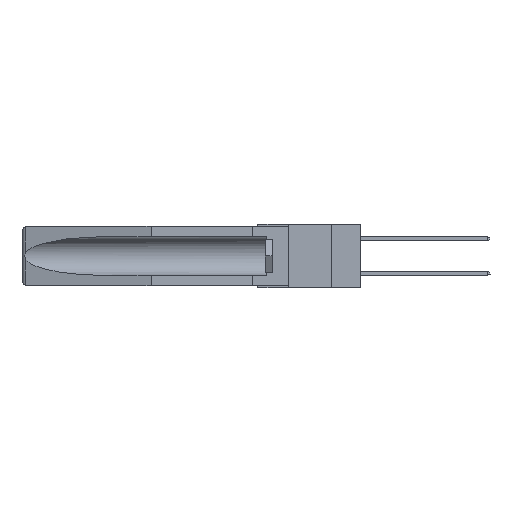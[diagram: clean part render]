
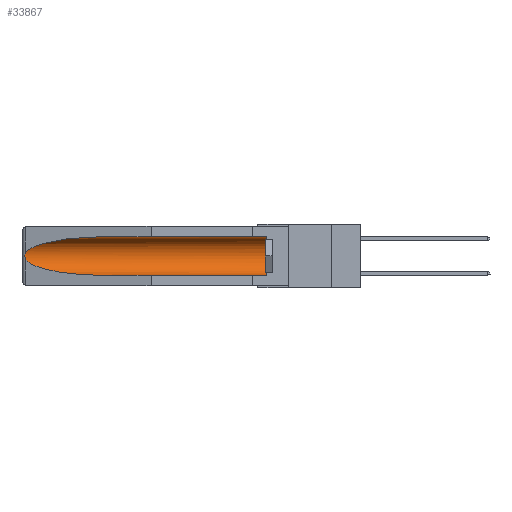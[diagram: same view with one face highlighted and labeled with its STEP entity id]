
A CAD part, left-side view. The second image highlights one B-rep face of the part: STEP entity #33867.
In plain terms, the highlighted cylindrical face has radius 2.857 mm (diameter 5.715 mm), a partial arc.
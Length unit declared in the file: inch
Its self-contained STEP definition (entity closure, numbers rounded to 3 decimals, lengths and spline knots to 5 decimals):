
#357 = ORIENTED_EDGE ( 'NONE', *, *, #7883, .T. ) ;
#951 = CARTESIAN_POINT ( 'NONE',  ( 0.26597, 1.5296, -0.19026 ) ) ;
#2775 = VERTEX_POINT ( 'NONE', #9192 ) ;
#3406 = EDGE_CURVE ( 'NONE', #28417, #9342, #11051, .T. ) ;
#3568 = CARTESIAN_POINT ( 'NONE',  ( 0.25451, 1.48313, -0.24835 ) ) ;
#3926 = DIRECTION ( 'NONE',  ( 0., 1., 0. ) ) ;
#4068 = ORIENTED_EDGE ( 'NONE', *, *, #5181, .T. ) ;
#4510 = AXIS2_PLACEMENT_3D ( 'NONE', #30480, #3926, #11827 ) ;
#4662 = CARTESIAN_POINT ( 'NONE',  ( 0.26537, 1.52718, -0.14972 ) ) ;
#5181 = EDGE_CURVE ( 'NONE', #28417, #31468, #23787, .T. ) ;
#6007 = DIRECTION ( 'NONE',  ( 0., 1., 0. ) ) ;
#6482 = CARTESIAN_POINT ( 'NONE',  ( 0.26537, 1.52718, -0.14972 ) ) ;
#6804 = CARTESIAN_POINT ( 'NONE',  ( 0.155, -0.30754, -0.284 ) ) ;
#7494 = FACE_OUTER_BOUND ( 'NONE', #24996, .T. ) ;
#7732 = ORIENTED_EDGE ( 'NONE', *, *, #31549, .T. ) ;
#7883 = EDGE_CURVE ( 'NONE', #24285, #2775, #11555, .T. ) ;
#8576 = CARTESIAN_POINT ( 'NONE',  ( 0.155, 0.126, -0.1715 ) ) ;
#9192 = CARTESIAN_POINT ( 'NONE',  ( 0.26537, 1.52718, -0.19328 ) ) ;
#9342 = VERTEX_POINT ( 'NONE', #11975 ) ;
#9935 = EDGE_CURVE ( 'NONE', #2775, #9342, #34099, .T. ) ;
#11051 = LINE ( 'NONE', #6804, #15234 ) ;
#11555 = B_SPLINE_CURVE_WITH_KNOTS ( 'NONE', 3,
 ( #6482, #22563, #30029, #14209, #14314, #32704, #19644, #16861, #951, #25066 ),
 .UNSPECIFIED., .F., .F.,
 ( 4, 2, 2, 2, 4 ),
 ( 0., 0.00029, 0.00058, 0.00087, 0.00117 ),
 .UNSPECIFIED. ) ;
#11804 = CARTESIAN_POINT ( 'NONE',  ( 0.26537, 1.52718, -0.19328 ) ) ;
#11827 = DIRECTION ( 'NONE',  ( 0., 0., 1. ) ) ;
#11975 = CARTESIAN_POINT ( 'NONE',  ( 0.155, 1.07973, -0.284 ) ) ;
#14209 = CARTESIAN_POINT ( 'NONE',  ( 0.2673, 1.5327, -0.16383 ) ) ;
#14314 = CARTESIAN_POINT ( 'NONE',  ( 0.2675, 1.53308, -0.16763 ) ) ;
#15201 =( BOUNDED_CURVE ( )  B_SPLINE_CURVE ( 3, ( #15371, #20609, #15599, #4662 ),
 .UNSPECIFIED., .F., .T. ) 
 B_SPLINE_CURVE_WITH_KNOTS ( ( 4, 4 ),
 ( 4.71239, 6.08839 ),
 .UNSPECIFIED. ) 
 CURVE ( )  GEOMETRIC_REPRESENTATION_ITEM ( )  RATIONAL_B_SPLINE_CURVE ( ( 1., 0.848, 0.848, 1. ) ) 
 REPRESENTATION_ITEM ( '' )  );
#15234 = VECTOR ( 'NONE', #19861, 39.37008 ) ;
#15371 = CARTESIAN_POINT ( 'NONE',  ( 0.155, 1.07973, -0.059 ) ) ;
#15599 = CARTESIAN_POINT ( 'NONE',  ( 0.25451, 1.48313, -0.09465 ) ) ;
#16861 = CARTESIAN_POINT ( 'NONE',  ( 0.26655, 1.53094, -0.18657 ) ) ;
#17263 = ORIENTED_EDGE ( 'NONE', *, *, #28318, .T. ) ;
#19644 = CARTESIAN_POINT ( 'NONE',  ( 0.2673, 1.53269, -0.17917 ) ) ;
#19861 = DIRECTION ( 'NONE',  ( 0., 1., 0. ) ) ;
#20609 = CARTESIAN_POINT ( 'NONE',  ( 0.21114, 1.30732, -0.059 ) ) ;
#20952 = LINE ( 'NONE', #27041, #21342 ) ;
#21342 = VECTOR ( 'NONE', #6007, 39.37008 ) ;
#21352 = ORIENTED_EDGE ( 'NONE', *, *, #9935, .T. ) ;
#22077 = DIRECTION ( 'NONE',  ( 0., 0., 1. ) ) ;
#22522 = CARTESIAN_POINT ( 'NONE',  ( 0.155, 1.07973, -0.284 ) ) ;
#22563 = CARTESIAN_POINT ( 'NONE',  ( 0.26597, 1.52961, -0.15275 ) ) ;
#23336 = AXIS2_PLACEMENT_3D ( 'NONE', #8576, #27131, #22077 ) ;
#23527 = CARTESIAN_POINT ( 'NONE',  ( 0.155, 1.07973, -0.059 ) ) ;
#23596 = CARTESIAN_POINT ( 'NONE',  ( 0.26537, 1.52718, -0.14972 ) ) ;
#23787 = CIRCLE ( 'NONE', #23336, 0.1125 ) ;
#24285 = VERTEX_POINT ( 'NONE', #23596 ) ;
#24996 = EDGE_LOOP ( 'NONE', ( #7732, #357, #21352, #26945, #4068, #17263 ) ) ;
#25066 = CARTESIAN_POINT ( 'NONE',  ( 0.26537, 1.52718, -0.19328 ) ) ;
#26945 = ORIENTED_EDGE ( 'NONE', *, *, #3406, .F. ) ;
#27041 = CARTESIAN_POINT ( 'NONE',  ( 0.155, -0.30754, -0.059 ) ) ;
#27131 = DIRECTION ( 'NONE',  ( 0., -1., 0. ) ) ;
#28318 = EDGE_CURVE ( 'NONE', #31468, #32822, #20952, .T. ) ;
#28417 = VERTEX_POINT ( 'NONE', #30015 ) ;
#30015 = CARTESIAN_POINT ( 'NONE',  ( 0.155, 0.126, -0.284 ) ) ;
#30029 = CARTESIAN_POINT ( 'NONE',  ( 0.26654, 1.53092, -0.15636 ) ) ;
#30480 = CARTESIAN_POINT ( 'NONE',  ( 0.155, -0.30754, -0.1715 ) ) ;
#30519 = CARTESIAN_POINT ( 'NONE',  ( 0.155, 0.126, -0.059 ) ) ;
#31150 = CYLINDRICAL_SURFACE ( 'NONE', #4510, 0.1125 ) ;
#31468 = VERTEX_POINT ( 'NONE', #30519 ) ;
#31549 = EDGE_CURVE ( 'NONE', #32822, #24285, #15201, .T. ) ;
#32704 = CARTESIAN_POINT ( 'NONE',  ( 0.2675, 1.53308, -0.17534 ) ) ;
#32822 = VERTEX_POINT ( 'NONE', #23527 ) ;
#33016 = CARTESIAN_POINT ( 'NONE',  ( 0.21114, 1.30732, -0.284 ) ) ;
#33867 = ADVANCED_FACE ( 'NONE', ( #7494 ), #31150, .F. ) ;
#34099 =( BOUNDED_CURVE ( )  B_SPLINE_CURVE ( 3, ( #11804, #3568, #33016, #22522 ),
 .UNSPECIFIED., .F., .F. ) 
 B_SPLINE_CURVE_WITH_KNOTS ( ( 4, 4 ),
 ( 0.1948, 1.5708 ),
 .UNSPECIFIED. ) 
 CURVE ( )  GEOMETRIC_REPRESENTATION_ITEM ( )  RATIONAL_B_SPLINE_CURVE ( ( 1., 0.848, 0.848, 1. ) ) 
 REPRESENTATION_ITEM ( '' )  );
